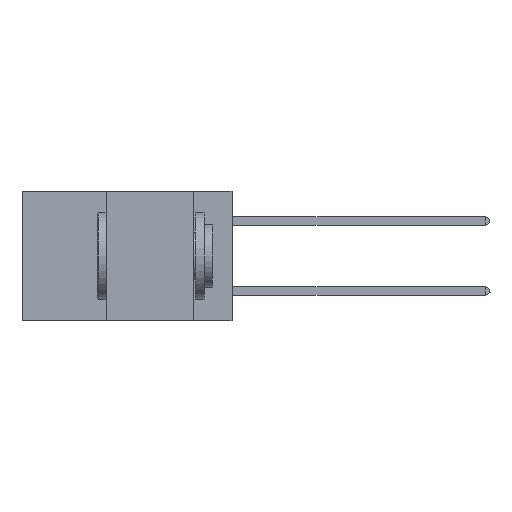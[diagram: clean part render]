
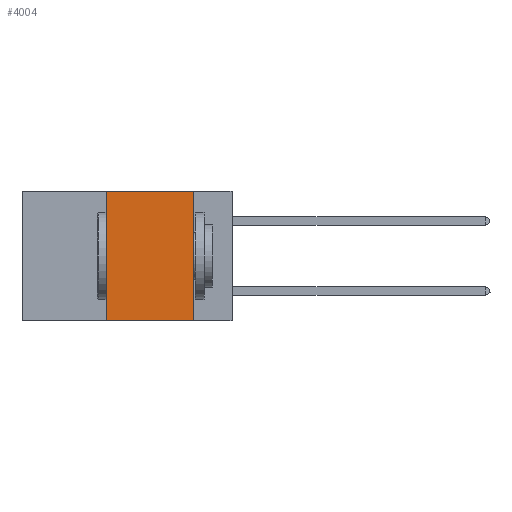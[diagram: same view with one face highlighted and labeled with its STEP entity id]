
A CAD part, left-side view. The second image highlights one B-rep face of the part: STEP entity #4004.
In plain terms, the highlighted planar face has unit normal (-1, 0, 0).
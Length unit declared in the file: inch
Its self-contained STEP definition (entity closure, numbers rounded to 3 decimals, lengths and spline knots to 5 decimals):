
#1157 = DIRECTION ( 'NONE',  ( 0., -1., 0. ) ) ;
#2385 = VERTEX_POINT ( 'NONE', #18336 ) ;
#3002 = VECTOR ( 'NONE', #13976, 39.37008 ) ;
#3238 = VECTOR ( 'NONE', #17776, 39.37008 ) ;
#3422 = DIRECTION ( 'NONE',  ( 0., 0., 1. ) ) ;
#3596 = ORIENTED_EDGE ( 'NONE', *, *, #10814, .F. ) ;
#3717 = CARTESIAN_POINT ( 'NONE',  ( 0., 0.6, 0. ) ) ;
#3965 = DIRECTION ( 'NONE',  ( 1., 0., 0. ) ) ;
#4004 = ADVANCED_FACE ( 'NONE', ( #18790 ), #7571, .F. ) ;
#4164 = EDGE_LOOP ( 'NONE', ( #12859, #3596, #12982, #7549 ) ) ;
#4387 = AXIS2_PLACEMENT_3D ( 'NONE', #14302, #3965, #9283 ) ;
#5341 = VERTEX_POINT ( 'NONE', #5937 ) ;
#5937 = CARTESIAN_POINT ( 'NONE',  ( 0., 0.36, -0.37 ) ) ;
#6133 = CARTESIAN_POINT ( 'NONE',  ( 0., 0.36, 0. ) ) ;
#7549 = ORIENTED_EDGE ( 'NONE', *, *, #21836, .T. ) ;
#7571 = PLANE ( 'NONE',  #4387 ) ;
#8125 = CARTESIAN_POINT ( 'NONE',  ( 0., 0.6, -0.37 ) ) ;
#9283 = DIRECTION ( 'NONE',  ( 0., 0., -1. ) ) ;
#9510 = LINE ( 'NONE', #13912, #16849 ) ;
#10043 = EDGE_CURVE ( 'NONE', #12541, #2385, #10115, .T. ) ;
#10115 = LINE ( 'NONE', #20694, #3002 ) ;
#10814 = EDGE_CURVE ( 'NONE', #21223, #12541, #11506, .T. ) ;
#11506 = LINE ( 'NONE', #3717, #3238 ) ;
#12009 = EDGE_CURVE ( 'NONE', #5341, #21223, #9510, .T. ) ;
#12541 = VERTEX_POINT ( 'NONE', #15887 ) ;
#12859 = ORIENTED_EDGE ( 'NONE', *, *, #10043, .F. ) ;
#12982 = ORIENTED_EDGE ( 'NONE', *, *, #12009, .F. ) ;
#12986 = LINE ( 'NONE', #8125, #20040 ) ;
#13912 = CARTESIAN_POINT ( 'NONE',  ( 0., 0.36, 0. ) ) ;
#13976 = DIRECTION ( 'NONE',  ( 0., 0., -1. ) ) ;
#14302 = CARTESIAN_POINT ( 'NONE',  ( 0., 0.6, 0. ) ) ;
#15887 = CARTESIAN_POINT ( 'NONE',  ( 0., 0.11, 0. ) ) ;
#16849 = VECTOR ( 'NONE', #3422, 39.37008 ) ;
#17776 = DIRECTION ( 'NONE',  ( 0., -1., 0. ) ) ;
#18336 = CARTESIAN_POINT ( 'NONE',  ( 0., 0.11, -0.37 ) ) ;
#18790 = FACE_OUTER_BOUND ( 'NONE', #4164, .T. ) ;
#20040 = VECTOR ( 'NONE', #1157, 39.37008 ) ;
#20694 = CARTESIAN_POINT ( 'NONE',  ( 0., 0.11, 0. ) ) ;
#21223 = VERTEX_POINT ( 'NONE', #6133 ) ;
#21836 = EDGE_CURVE ( 'NONE', #5341, #2385, #12986, .T. ) ;
